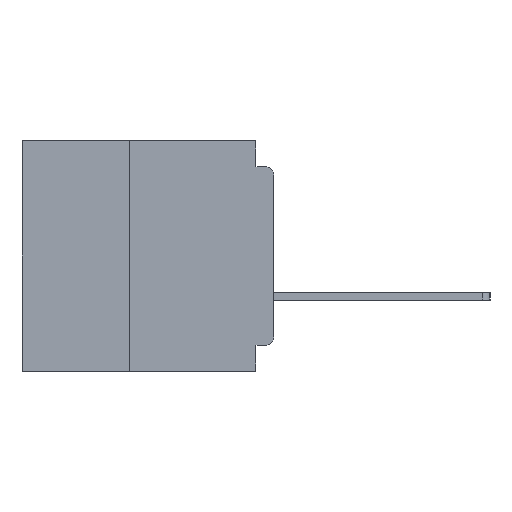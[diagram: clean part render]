
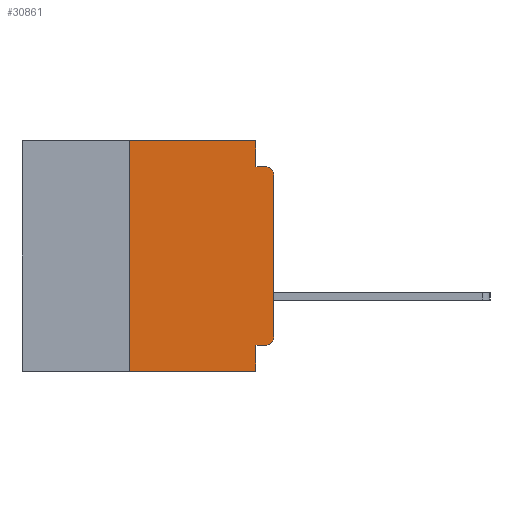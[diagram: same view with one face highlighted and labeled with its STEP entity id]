
A CAD part, left-side view. The second image highlights one B-rep face of the part: STEP entity #30861.
In plain terms, the highlighted planar face has unit normal (-1, 0, 0).
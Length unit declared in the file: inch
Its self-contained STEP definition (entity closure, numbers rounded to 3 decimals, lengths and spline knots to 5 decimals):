
#1750 = CARTESIAN_POINT ( 'NONE',  ( 0., 0.031, -0.355 ) ) ;
#2016 = EDGE_CURVE ( 'NONE', #22683, #39920, #6895, .T. ) ;
#2756 = CARTESIAN_POINT ( 'NONE',  ( 0., 0.437, 0. ) ) ;
#4955 = CARTESIAN_POINT ( 'NONE',  ( 0., 0.25, -0.4 ) ) ;
#5305 = VERTEX_POINT ( 'NONE', #40172 ) ;
#5616 = CARTESIAN_POINT ( 'NONE',  ( 0., 0.031, 0. ) ) ;
#5830 = ORIENTED_EDGE ( 'NONE', *, *, #2016, .F. ) ;
#6129 = PLANE ( 'NONE',  #19571 ) ;
#6663 = LINE ( 'NONE', #38075, #22439 ) ;
#6788 = EDGE_CURVE ( 'NONE', #5305, #10187, #37537, .T. ) ;
#6895 = LINE ( 'NONE', #10980, #26848 ) ;
#6953 = EDGE_CURVE ( 'NONE', #39920, #10740, #6663, .T. ) ;
#8340 = CARTESIAN_POINT ( 'NONE',  ( 0., 0.437, -0.4 ) ) ;
#8536 = ORIENTED_EDGE ( 'NONE', *, *, #37930, .T. ) ;
#8742 = ORIENTED_EDGE ( 'NONE', *, *, #22080, .T. ) ;
#9309 = DIRECTION ( 'NONE',  ( -1., 0., 0. ) ) ;
#9485 = DIRECTION ( 'NONE',  ( 0., 0., -1. ) ) ;
#10187 = VERTEX_POINT ( 'NONE', #12084 ) ;
#10740 = VERTEX_POINT ( 'NONE', #5616 ) ;
#10980 = CARTESIAN_POINT ( 'NONE',  ( 0., 0.25, -0.4 ) ) ;
#11249 = AXIS2_PLACEMENT_3D ( 'NONE', #14398, #37737, #17816 ) ;
#11294 = ORIENTED_EDGE ( 'NONE', *, *, #36842, .T. ) ;
#12084 = CARTESIAN_POINT ( 'NONE',  ( 0., 0.015, -0.045 ) ) ;
#12189 = CIRCLE ( 'NONE', #26729, 0.015 ) ;
#12593 = CARTESIAN_POINT ( 'NONE',  ( 0., 0., -0.355 ) ) ;
#14007 = ORIENTED_EDGE ( 'NONE', *, *, #6953, .F. ) ;
#14308 = LINE ( 'NONE', #12593, #31053 ) ;
#14398 = CARTESIAN_POINT ( 'NONE',  ( 0., 0.015, -0.34 ) ) ;
#15421 = DIRECTION ( 'NONE',  ( 0., 0., -1. ) ) ;
#15426 = VERTEX_POINT ( 'NONE', #29643 ) ;
#15993 = DIRECTION ( 'NONE',  ( 0., 1., 0. ) ) ;
#16516 = CIRCLE ( 'NONE', #11249, 0.015 ) ;
#17153 = VECTOR ( 'NONE', #28259, 39.37008 ) ;
#17324 = DIRECTION ( 'NONE',  ( 0., -1., 0. ) ) ;
#17392 = VECTOR ( 'NONE', #31768, 39.37008 ) ;
#17816 = DIRECTION ( 'NONE',  ( 0., 0., -1. ) ) ;
#18517 = CARTESIAN_POINT ( 'NONE',  ( 0., 0.031, -0.4 ) ) ;
#19571 = AXIS2_PLACEMENT_3D ( 'NONE', #2756, #42623, #9485 ) ;
#20942 = ORIENTED_EDGE ( 'NONE', *, *, #34422, .F. ) ;
#21427 = ORIENTED_EDGE ( 'NONE', *, *, #6788, .F. ) ;
#22080 = EDGE_CURVE ( 'NONE', #15426, #30247, #42563, .T. ) ;
#22439 = VECTOR ( 'NONE', #41420, 39.37008 ) ;
#22683 = VERTEX_POINT ( 'NONE', #4955 ) ;
#22815 = VERTEX_POINT ( 'NONE', #39086 ) ;
#24907 = VECTOR ( 'NONE', #32067, 39.37008 ) ;
#26008 = LINE ( 'NONE', #41452, #17153 ) ;
#26729 = AXIS2_PLACEMENT_3D ( 'NONE', #29385, #9309, #32714 ) ;
#26848 = VECTOR ( 'NONE', #27668, 39.37008 ) ;
#27668 = DIRECTION ( 'NONE',  ( 0., 0., 1. ) ) ;
#28259 = DIRECTION ( 'NONE',  ( 0., 0., -1. ) ) ;
#28347 = EDGE_CURVE ( 'NONE', #10740, #5305, #26008, .T. ) ;
#28702 = VECTOR ( 'NONE', #17324, 39.37008 ) ;
#29141 = CARTESIAN_POINT ( 'NONE',  ( 0., 0.25, 0. ) ) ;
#29385 = CARTESIAN_POINT ( 'NONE',  ( 0., 0.015, -0.06 ) ) ;
#29643 = CARTESIAN_POINT ( 'NONE',  ( 0., 0., -0.34 ) ) ;
#30247 = VERTEX_POINT ( 'NONE', #42961 ) ;
#30585 = CARTESIAN_POINT ( 'NONE',  ( 0., 0., -0.045 ) ) ;
#30861 = ADVANCED_FACE ( 'NONE', ( #35516 ), #6129, .F. ) ;
#31053 = VECTOR ( 'NONE', #15993, 39.37008 ) ;
#31768 = DIRECTION ( 'NONE',  ( 0., -1., 0. ) ) ;
#32067 = DIRECTION ( 'NONE',  ( 0., 0., 1. ) ) ;
#32577 = ORIENTED_EDGE ( 'NONE', *, *, #35897, .T. ) ;
#32714 = DIRECTION ( 'NONE',  ( 0., 0., -1. ) ) ;
#33248 = EDGE_LOOP ( 'NONE', ( #8742, #11294, #21427, #37986, #14007, #5830, #8536, #36871, #20942, #32577 ) ) ;
#33324 = EDGE_CURVE ( 'NONE', #40573, #36036, #39433, .T. ) ;
#34422 = EDGE_CURVE ( 'NONE', #22815, #40573, #14308, .T. ) ;
#35380 = CARTESIAN_POINT ( 'NONE',  ( 0., 0., 0. ) ) ;
#35516 = FACE_OUTER_BOUND ( 'NONE', #33248, .T. ) ;
#35897 = EDGE_CURVE ( 'NONE', #22815, #15426, #16516, .T. ) ;
#36036 = VERTEX_POINT ( 'NONE', #18517 ) ;
#36842 = EDGE_CURVE ( 'NONE', #30247, #10187, #12189, .T. ) ;
#36871 = ORIENTED_EDGE ( 'NONE', *, *, #33324, .F. ) ;
#37179 = LINE ( 'NONE', #8340, #17392 ) ;
#37537 = LINE ( 'NONE', #30585, #28702 ) ;
#37737 = DIRECTION ( 'NONE',  ( -1., 0., 0. ) ) ;
#37930 = EDGE_CURVE ( 'NONE', #22683, #36036, #37179, .T. ) ;
#37986 = ORIENTED_EDGE ( 'NONE', *, *, #28347, .F. ) ;
#38075 = CARTESIAN_POINT ( 'NONE',  ( 0., 0.437, 0. ) ) ;
#38732 = CARTESIAN_POINT ( 'NONE',  ( 0., 0.031, -0.4 ) ) ;
#39086 = CARTESIAN_POINT ( 'NONE',  ( 0., 0.015, -0.355 ) ) ;
#39433 = LINE ( 'NONE', #38732, #40502 ) ;
#39920 = VERTEX_POINT ( 'NONE', #29141 ) ;
#40172 = CARTESIAN_POINT ( 'NONE',  ( 0., 0.031, -0.045 ) ) ;
#40502 = VECTOR ( 'NONE', #15421, 39.37008 ) ;
#40573 = VERTEX_POINT ( 'NONE', #1750 ) ;
#41420 = DIRECTION ( 'NONE',  ( 0., -1., 0. ) ) ;
#41452 = CARTESIAN_POINT ( 'NONE',  ( 0., 0.031, 0. ) ) ;
#42563 = LINE ( 'NONE', #35380, #24907 ) ;
#42623 = DIRECTION ( 'NONE',  ( 1., 0., 0. ) ) ;
#42961 = CARTESIAN_POINT ( 'NONE',  ( 0., 0., -0.06 ) ) ;
